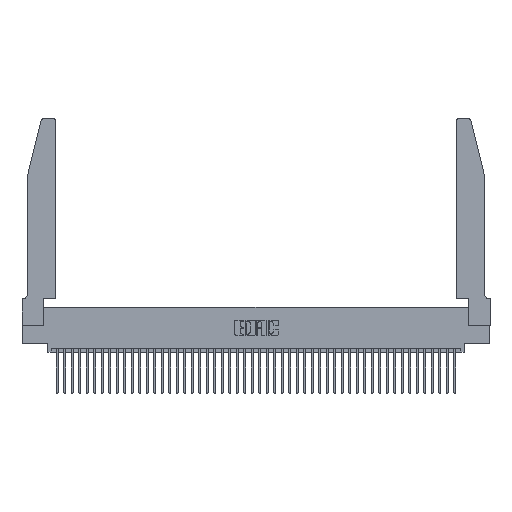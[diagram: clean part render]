
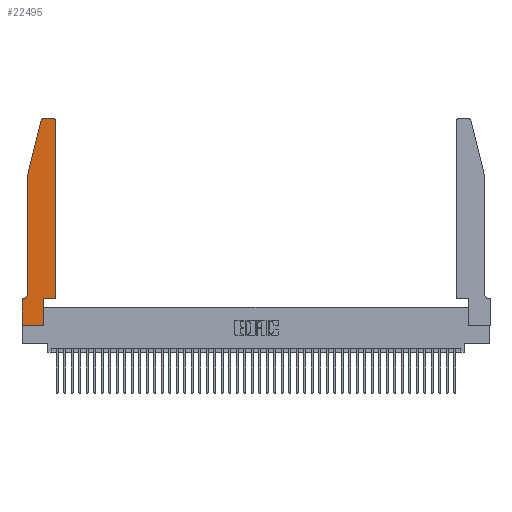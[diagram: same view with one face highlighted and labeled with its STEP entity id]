
A CAD part, top view. The second image highlights one B-rep face of the part: STEP entity #22495.
In plain terms, the highlighted planar face has unit normal (0, 0, 1).
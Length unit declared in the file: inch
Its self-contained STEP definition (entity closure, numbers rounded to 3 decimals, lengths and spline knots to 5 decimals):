
#1 = DIRECTION ( 'NONE',  ( -1., 0., 0. ) ) ;
#158 = DIRECTION ( 'NONE',  ( -1., 0., 0. ) ) ;
#1341 = VERTEX_POINT ( 'NONE', #11534 ) ;
#2040 = VERTEX_POINT ( 'NONE', #27339 ) ;
#2211 = AXIS2_PLACEMENT_3D ( 'NONE', #12408, #44006, #26425 ) ;
#3437 = VERTEX_POINT ( 'NONE', #13423 ) ;
#3588 = ORIENTED_EDGE ( 'NONE', *, *, #23891, .T. ) ;
#3947 = CARTESIAN_POINT ( 'NONE',  ( 0., 0., 0.37 ) ) ;
#4922 = VERTEX_POINT ( 'NONE', #28355 ) ;
#5412 = VECTOR ( 'NONE', #24467, 39.37008 ) ;
#7018 = EDGE_CURVE ( 'NONE', #19035, #22443, #40874, .T. ) ;
#7793 = CARTESIAN_POINT ( 'NONE',  ( 0.4205, 2.75, 0.37 ) ) ;
#8053 = CARTESIAN_POINT ( 'NONE',  ( 0.0055, 0.35, 0.37 ) ) ;
#8437 = AXIS2_PLACEMENT_3D ( 'NONE', #42694, #43303, #35929 ) ;
#8492 = VERTEX_POINT ( 'NONE', #11226 ) ;
#9961 = PLANE ( 'NONE',  #11337 ) ;
#11226 = CARTESIAN_POINT ( 'NONE',  ( 0.2865, 0.35, 0.37 ) ) ;
#11337 = AXIS2_PLACEMENT_3D ( 'NONE', #27673, #17369, #42013 ) ;
#11534 = CARTESIAN_POINT ( 'NONE',  ( 0., 0., 0.37 ) ) ;
#12206 = VECTOR ( 'NONE', #45564, 39.37008 ) ;
#12292 = EDGE_CURVE ( 'NONE', #3437, #8492, #39923, .T. ) ;
#12314 = VECTOR ( 'NONE', #28136, 39.37008 ) ;
#12408 = CARTESIAN_POINT ( 'NONE',  ( 0.4205, 2.72, 0.37 ) ) ;
#13423 = CARTESIAN_POINT ( 'NONE',  ( 0.2865, 0., 0.37 ) ) ;
#13746 = DIRECTION ( 'NONE',  ( -0.239, -0.971, 0. ) ) ;
#13832 = DIRECTION ( 'NONE',  ( 0., 0., 1. ) ) ;
#14026 = CARTESIAN_POINT ( 'NONE',  ( 0.4505, 0.35, 0.37 ) ) ;
#14155 = CARTESIAN_POINT ( 'NONE',  ( 0.0755, 2., 0.37 ) ) ;
#14284 = ORIENTED_EDGE ( 'NONE', *, *, #12292, .T. ) ;
#15241 = DIRECTION ( 'NONE',  ( 0., -1., 0. ) ) ;
#15421 = DIRECTION ( 'NONE',  ( 1., 0., 0. ) ) ;
#17159 = VECTOR ( 'NONE', #15241, 39.37008 ) ;
#17307 = EDGE_CURVE ( 'NONE', #8492, #19035, #39821, .T. ) ;
#17369 = DIRECTION ( 'NONE',  ( 0., 0., 1. ) ) ;
#17510 = VECTOR ( 'NONE', #158, 39.37008 ) ;
#17661 = CARTESIAN_POINT ( 'NONE',  ( 0.4505, 2.72, 0.37 ) ) ;
#17923 = CARTESIAN_POINT ( 'NONE',  ( 0.0755, 0.35, 0.37 ) ) ;
#18701 = ORIENTED_EDGE ( 'NONE', *, *, #26413, .T. ) ;
#19035 = VERTEX_POINT ( 'NONE', #14026 ) ;
#19174 = EDGE_LOOP ( 'NONE', ( #39214, #18701, #41348, #3588, #36812, #25841, #34225, #32055, #14284, #32662, #19594, #20483 ) ) ;
#19594 = ORIENTED_EDGE ( 'NONE', *, *, #7018, .T. ) ;
#20450 = VECTOR ( 'NONE', #1, 39.37008 ) ;
#20483 = ORIENTED_EDGE ( 'NONE', *, *, #34603, .T. ) ;
#21347 = CARTESIAN_POINT ( 'NONE',  ( 0.0755, 2., 0.37 ) ) ;
#22443 = VERTEX_POINT ( 'NONE', #17661 ) ;
#22495 = ADVANCED_FACE ( 'NONE', ( #40899 ), #9961, .T. ) ;
#22617 = LINE ( 'NONE', #24668, #20450 ) ;
#23166 = EDGE_CURVE ( 'NONE', #45027, #4922, #22617, .T. ) ;
#23891 = EDGE_CURVE ( 'NONE', #42892, #35407, #40738, .T. ) ;
#24362 = VECTOR ( 'NONE', #15421, 39.37008 ) ;
#24467 = DIRECTION ( 'NONE',  ( 0., -1., 0. ) ) ;
#24640 = LINE ( 'NONE', #17923, #17510 ) ;
#24668 = CARTESIAN_POINT ( 'NONE',  ( 0.2605, 2.75, 0.37 ) ) ;
#24687 = AXIS2_PLACEMENT_3D ( 'NONE', #42317, #13832, #35103 ) ;
#24742 = CARTESIAN_POINT ( 'NONE',  ( 0.4505, 0.35, 0.37 ) ) ;
#25372 = CARTESIAN_POINT ( 'NONE',  ( 0., 0.35, 0.37 ) ) ;
#25841 = ORIENTED_EDGE ( 'NONE', *, *, #31970, .T. ) ;
#26413 = EDGE_CURVE ( 'NONE', #4922, #2040, #33954, .T. ) ;
#26425 = DIRECTION ( 'NONE',  ( 1., 0., 0. ) ) ;
#26547 = VECTOR ( 'NONE', #42209, 39.37008 ) ;
#27046 = LINE ( 'NONE', #35736, #17159 ) ;
#27339 = CARTESIAN_POINT ( 'NONE',  ( 0.25487, 2.72718, 0.37 ) ) ;
#27673 = CARTESIAN_POINT ( 'NONE',  ( 0., 0.35, 0.37 ) ) ;
#28136 = DIRECTION ( 'NONE',  ( 0., 1., 0. ) ) ;
#28355 = CARTESIAN_POINT ( 'NONE',  ( 0.284, 2.75, 0.37 ) ) ;
#29654 = CARTESIAN_POINT ( 'NONE',  ( 0.0755, 0.42, 0.37 ) ) ;
#30029 = EDGE_CURVE ( 'NONE', #36761, #1341, #27046, .T. ) ;
#30292 = LINE ( 'NONE', #31357, #40194 ) ;
#31100 = EDGE_CURVE ( 'NONE', #2040, #42892, #30292, .T. ) ;
#31357 = CARTESIAN_POINT ( 'NONE',  ( 0.0755, 2., 0.37 ) ) ;
#31565 = CARTESIAN_POINT ( 'NONE',  ( 0.2865, 0.35, 0.37 ) ) ;
#31970 = EDGE_CURVE ( 'NONE', #35196, #36761, #24640, .T. ) ;
#32055 = ORIENTED_EDGE ( 'NONE', *, *, #44767, .T. ) ;
#32662 = ORIENTED_EDGE ( 'NONE', *, *, #17307, .T. ) ;
#32998 = CARTESIAN_POINT ( 'NONE',  ( 0.4505, 0.35, 0.37 ) ) ;
#33225 = LINE ( 'NONE', #3947, #26547 ) ;
#33954 = CIRCLE ( 'NONE', #24687, 0.03 ) ;
#34225 = ORIENTED_EDGE ( 'NONE', *, *, #30029, .T. ) ;
#34603 = EDGE_CURVE ( 'NONE', #22443, #45027, #37760, .T. ) ;
#35103 = DIRECTION ( 'NONE',  ( 1., 0., 0. ) ) ;
#35196 = VERTEX_POINT ( 'NONE', #8053 ) ;
#35407 = VERTEX_POINT ( 'NONE', #29654 ) ;
#35736 = CARTESIAN_POINT ( 'NONE',  ( 0., 0., 0.37 ) ) ;
#35929 = DIRECTION ( 'NONE',  ( -1., 0., 0. ) ) ;
#36111 = EDGE_CURVE ( 'NONE', #35407, #35196, #38155, .T. ) ;
#36761 = VERTEX_POINT ( 'NONE', #25372 ) ;
#36812 = ORIENTED_EDGE ( 'NONE', *, *, #36111, .T. ) ;
#37760 = CIRCLE ( 'NONE', #2211, 0.03 ) ;
#38155 = CIRCLE ( 'NONE', #8437, 0.07 ) ;
#39214 = ORIENTED_EDGE ( 'NONE', *, *, #23166, .T. ) ;
#39821 = LINE ( 'NONE', #32998, #24362 ) ;
#39923 = LINE ( 'NONE', #31565, #12314 ) ;
#40194 = VECTOR ( 'NONE', #13746, 39.37008 ) ;
#40738 = LINE ( 'NONE', #14155, #5412 ) ;
#40874 = LINE ( 'NONE', #24742, #12206 ) ;
#40899 = FACE_OUTER_BOUND ( 'NONE', #19174, .T. ) ;
#41348 = ORIENTED_EDGE ( 'NONE', *, *, #31100, .T. ) ;
#42013 = DIRECTION ( 'NONE',  ( 1., 0., 0. ) ) ;
#42209 = DIRECTION ( 'NONE',  ( 1., 0., 0. ) ) ;
#42317 = CARTESIAN_POINT ( 'NONE',  ( 0.284, 2.72, 0.37 ) ) ;
#42694 = CARTESIAN_POINT ( 'NONE',  ( 0.0055, 0.42, 0.37 ) ) ;
#42892 = VERTEX_POINT ( 'NONE', #21347 ) ;
#43303 = DIRECTION ( 'NONE',  ( 0., 0., -1. ) ) ;
#44006 = DIRECTION ( 'NONE',  ( 0., 0., 1. ) ) ;
#44767 = EDGE_CURVE ( 'NONE', #1341, #3437, #33225, .T. ) ;
#45027 = VERTEX_POINT ( 'NONE', #7793 ) ;
#45564 = DIRECTION ( 'NONE',  ( 0., 1., 0. ) ) ;
